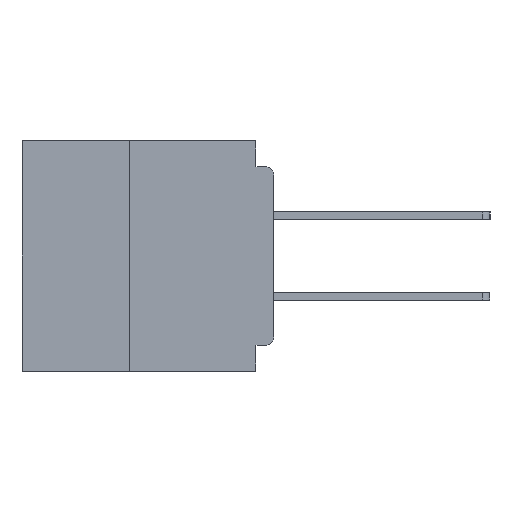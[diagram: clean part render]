
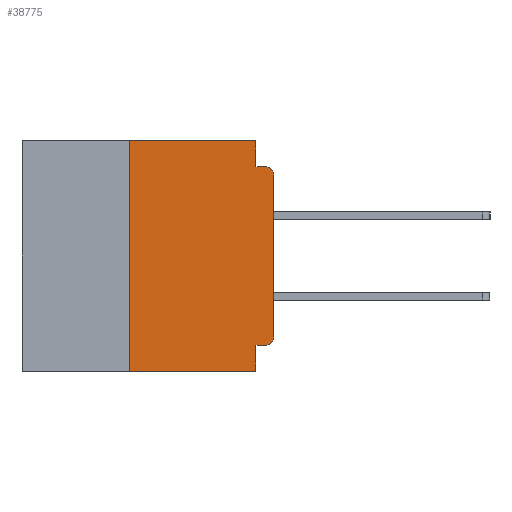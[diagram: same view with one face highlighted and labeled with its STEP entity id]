
A CAD part, left-side view. The second image highlights one B-rep face of the part: STEP entity #38775.
In plain terms, the highlighted planar face has unit normal (-1, 0, 0).
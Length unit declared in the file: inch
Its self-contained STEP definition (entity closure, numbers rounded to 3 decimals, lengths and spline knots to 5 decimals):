
#201 = ORIENTED_EDGE ( 'NONE', *, *, #36335, .T. ) ;
#1334 = CARTESIAN_POINT ( 'NONE',  ( 0., 0., -0.355 ) ) ;
#2488 = EDGE_CURVE ( 'NONE', #3869, #3450, #18583, .T. ) ;
#2996 = CARTESIAN_POINT ( 'NONE',  ( 0., 0.25, 0. ) ) ;
#3439 = PLANE ( 'NONE',  #36135 ) ;
#3450 = VERTEX_POINT ( 'NONE', #18117 ) ;
#3869 = VERTEX_POINT ( 'NONE', #2996 ) ;
#4050 = CARTESIAN_POINT ( 'NONE',  ( 0., 0.015, -0.355 ) ) ;
#5151 = ORIENTED_EDGE ( 'NONE', *, *, #34442, .T. ) ;
#5527 = VERTEX_POINT ( 'NONE', #12122 ) ;
#5582 = CARTESIAN_POINT ( 'NONE',  ( 0., 0.015, -0.045 ) ) ;
#5886 = VECTOR ( 'NONE', #10750, 39.37008 ) ;
#6623 = DIRECTION ( 'NONE',  ( 1., 0., 0. ) ) ;
#6934 = VECTOR ( 'NONE', #19863, 39.37008 ) ;
#7153 = LINE ( 'NONE', #35845, #15316 ) ;
#7208 = ORIENTED_EDGE ( 'NONE', *, *, #7904, .F. ) ;
#7431 = CARTESIAN_POINT ( 'NONE',  ( 0., 0., -0.34 ) ) ;
#7520 = EDGE_LOOP ( 'NONE', ( #201, #5151, #7208, #8670, #9462, #9621, #12710, #15407, #19531, #19955 ) ) ;
#7588 = CARTESIAN_POINT ( 'NONE',  ( 0., 0., -0.045 ) ) ;
#7904 = EDGE_CURVE ( 'NONE', #23866, #14811, #15088, .T. ) ;
#8556 = CARTESIAN_POINT ( 'NONE',  ( 0., 0.031, -0.045 ) ) ;
#8609 = VECTOR ( 'NONE', #21454, 39.37008 ) ;
#8670 = ORIENTED_EDGE ( 'NONE', *, *, #28306, .F. ) ;
#9462 = ORIENTED_EDGE ( 'NONE', *, *, #2488, .F. ) ;
#9621 = ORIENTED_EDGE ( 'NONE', *, *, #28360, .F. ) ;
#10230 = EDGE_CURVE ( 'NONE', #5527, #12161, #37316, .T. ) ;
#10539 = LINE ( 'NONE', #15373, #8609 ) ;
#10750 = DIRECTION ( 'NONE',  ( 0., 1., 0. ) ) ;
#12122 = CARTESIAN_POINT ( 'NONE',  ( 0., 0.031, -0.355 ) ) ;
#12161 = VERTEX_POINT ( 'NONE', #24001 ) ;
#12710 = ORIENTED_EDGE ( 'NONE', *, *, #18339, .T. ) ;
#13423 = AXIS2_PLACEMENT_3D ( 'NONE', #14413, #35339, #17478 ) ;
#13901 = LINE ( 'NONE', #31994, #19109 ) ;
#14413 = CARTESIAN_POINT ( 'NONE',  ( 0., 0.015, -0.34 ) ) ;
#14811 = VERTEX_POINT ( 'NONE', #5582 ) ;
#15083 = DIRECTION ( 'NONE',  ( 0., 0., 1. ) ) ;
#15088 = LINE ( 'NONE', #7588, #6934 ) ;
#15316 = VECTOR ( 'NONE', #18014, 39.37008 ) ;
#15373 = CARTESIAN_POINT ( 'NONE',  ( 0., 0., 0. ) ) ;
#15407 = ORIENTED_EDGE ( 'NONE', *, *, #10230, .F. ) ;
#16138 = CARTESIAN_POINT ( 'NONE',  ( 0., 0.015, -0.06 ) ) ;
#16510 = EDGE_CURVE ( 'NONE', #28106, #5527, #22101, .T. ) ;
#17017 = CARTESIAN_POINT ( 'NONE',  ( 0., 0., -0.06 ) ) ;
#17413 = CIRCLE ( 'NONE', #23758, 0.015 ) ;
#17429 = DIRECTION ( 'NONE',  ( 0., 0., -1. ) ) ;
#17478 = DIRECTION ( 'NONE',  ( 0., 0., -1. ) ) ;
#17545 = FACE_OUTER_BOUND ( 'NONE', #7520, .T. ) ;
#17791 = EDGE_CURVE ( 'NONE', #28106, #20983, #32759, .T. ) ;
#18014 = DIRECTION ( 'NONE',  ( 0., 0., -1. ) ) ;
#18117 = CARTESIAN_POINT ( 'NONE',  ( 0., 0.031, 0. ) ) ;
#18339 = EDGE_CURVE ( 'NONE', #26682, #12161, #13901, .T. ) ;
#18583 = LINE ( 'NONE', #33488, #26629 ) ;
#19109 = VECTOR ( 'NONE', #25988, 39.37008 ) ;
#19163 = DIRECTION ( 'NONE',  ( 0., 0., -1. ) ) ;
#19531 = ORIENTED_EDGE ( 'NONE', *, *, #16510, .F. ) ;
#19863 = DIRECTION ( 'NONE',  ( 0., -1., 0. ) ) ;
#19955 = ORIENTED_EDGE ( 'NONE', *, *, #17791, .T. ) ;
#20329 = CARTESIAN_POINT ( 'NONE',  ( 0., 0.031, -0.4 ) ) ;
#20983 = VERTEX_POINT ( 'NONE', #7431 ) ;
#21454 = DIRECTION ( 'NONE',  ( 0., 0., 1. ) ) ;
#21465 = VECTOR ( 'NONE', #15083, 39.37008 ) ;
#22101 = LINE ( 'NONE', #1334, #5886 ) ;
#23758 = AXIS2_PLACEMENT_3D ( 'NONE', #16138, #36942, #19163 ) ;
#23866 = VERTEX_POINT ( 'NONE', #8556 ) ;
#24001 = CARTESIAN_POINT ( 'NONE',  ( 0., 0.031, -0.4 ) ) ;
#24813 = CARTESIAN_POINT ( 'NONE',  ( 0., 0.437, 0. ) ) ;
#25988 = DIRECTION ( 'NONE',  ( 0., -1., 0. ) ) ;
#26629 = VECTOR ( 'NONE', #32992, 39.37008 ) ;
#26682 = VERTEX_POINT ( 'NONE', #29735 ) ;
#27830 = DIRECTION ( 'NONE',  ( 0., 0., -1. ) ) ;
#28106 = VERTEX_POINT ( 'NONE', #4050 ) ;
#28306 = EDGE_CURVE ( 'NONE', #3450, #23866, #7153, .T. ) ;
#28360 = EDGE_CURVE ( 'NONE', #26682, #3869, #29473, .T. ) ;
#29455 = VERTEX_POINT ( 'NONE', #17017 ) ;
#29473 = LINE ( 'NONE', #35964, #21465 ) ;
#29597 = VECTOR ( 'NONE', #17429, 39.37008 ) ;
#29735 = CARTESIAN_POINT ( 'NONE',  ( 0., 0.25, -0.4 ) ) ;
#31994 = CARTESIAN_POINT ( 'NONE',  ( 0., 0.437, -0.4 ) ) ;
#32759 = CIRCLE ( 'NONE', #13423, 0.015 ) ;
#32992 = DIRECTION ( 'NONE',  ( 0., -1., 0. ) ) ;
#33488 = CARTESIAN_POINT ( 'NONE',  ( 0., 0.437, 0. ) ) ;
#34442 = EDGE_CURVE ( 'NONE', #29455, #14811, #17413, .T. ) ;
#35339 = DIRECTION ( 'NONE',  ( -1., 0., 0. ) ) ;
#35845 = CARTESIAN_POINT ( 'NONE',  ( 0., 0.031, 0. ) ) ;
#35964 = CARTESIAN_POINT ( 'NONE',  ( 0., 0.25, -0.4 ) ) ;
#36135 = AXIS2_PLACEMENT_3D ( 'NONE', #24813, #6623, #27830 ) ;
#36335 = EDGE_CURVE ( 'NONE', #20983, #29455, #10539, .T. ) ;
#36942 = DIRECTION ( 'NONE',  ( -1., 0., 0. ) ) ;
#37316 = LINE ( 'NONE', #20329, #29597 ) ;
#38775 = ADVANCED_FACE ( 'NONE', ( #17545 ), #3439, .F. ) ;
